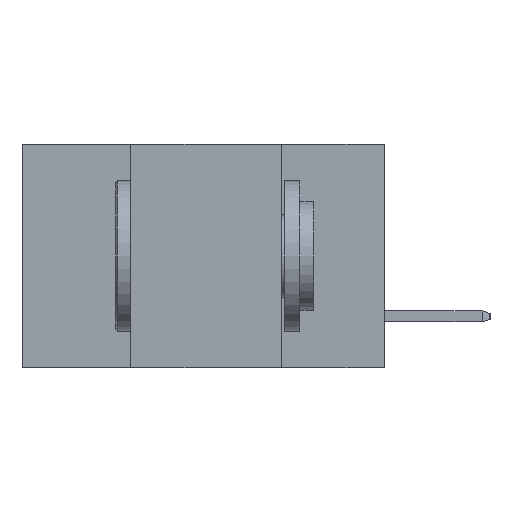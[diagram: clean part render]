
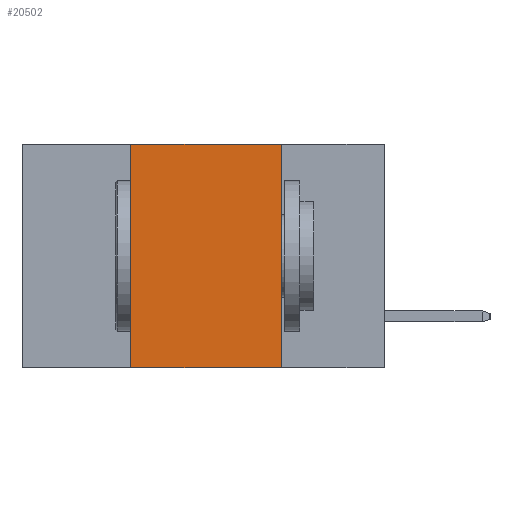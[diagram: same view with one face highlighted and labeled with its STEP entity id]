
A CAD part, left-side view. The second image highlights one B-rep face of the part: STEP entity #20502.
In plain terms, the highlighted planar face has unit normal (-1, 0, 0).
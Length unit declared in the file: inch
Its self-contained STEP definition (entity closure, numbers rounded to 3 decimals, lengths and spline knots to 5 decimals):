
#30 = DIRECTION ( 'NONE',  ( 0., 0., -1. ) ) ;
#224 = DIRECTION ( 'NONE',  ( 0., 0., 1. ) ) ;
#1218 = CARTESIAN_POINT ( 'NONE',  ( 0., 0.6, -0.37 ) ) ;
#2564 = LINE ( 'NONE', #15857, #6659 ) ;
#3887 = VERTEX_POINT ( 'NONE', #10185 ) ;
#6037 = EDGE_CURVE ( 'NONE', #11460, #7524, #2564, .T. ) ;
#6247 = CARTESIAN_POINT ( 'NONE',  ( 0., 0.17, -0.37 ) ) ;
#6659 = VECTOR ( 'NONE', #30, 39.37008 ) ;
#6867 = LINE ( 'NONE', #1218, #12126 ) ;
#7206 = ORIENTED_EDGE ( 'NONE', *, *, #8385, .F. ) ;
#7524 = VERTEX_POINT ( 'NONE', #6247 ) ;
#7824 = LINE ( 'NONE', #20864, #16975 ) ;
#8385 = EDGE_CURVE ( 'NONE', #17802, #11460, #7824, .T. ) ;
#9346 = DIRECTION ( 'NONE',  ( 0., -1., 0. ) ) ;
#10185 = CARTESIAN_POINT ( 'NONE',  ( 0., 0.42, -0.37 ) ) ;
#10246 = CARTESIAN_POINT ( 'NONE',  ( 0., 0.42, 0. ) ) ;
#11330 = FACE_OUTER_BOUND ( 'NONE', #12902, .T. ) ;
#11460 = VERTEX_POINT ( 'NONE', #13643 ) ;
#11835 = DIRECTION ( 'NONE',  ( 1., 0., 0. ) ) ;
#12126 = VECTOR ( 'NONE', #22686, 39.37008 ) ;
#12902 = EDGE_LOOP ( 'NONE', ( #16998, #7206, #14887, #19045 ) ) ;
#13643 = CARTESIAN_POINT ( 'NONE',  ( 0., 0.17, 0. ) ) ;
#14887 = ORIENTED_EDGE ( 'NONE', *, *, #24316, .F. ) ;
#15387 = VECTOR ( 'NONE', #224, 39.37008 ) ;
#15857 = CARTESIAN_POINT ( 'NONE',  ( 0., 0.17, 0. ) ) ;
#16975 = VECTOR ( 'NONE', #9346, 39.37008 ) ;
#16998 = ORIENTED_EDGE ( 'NONE', *, *, #6037, .F. ) ;
#17802 = VERTEX_POINT ( 'NONE', #18505 ) ;
#18505 = CARTESIAN_POINT ( 'NONE',  ( 0., 0.42, 0. ) ) ;
#18573 = AXIS2_PLACEMENT_3D ( 'NONE', #23291, #11835, #25206 ) ;
#19045 = ORIENTED_EDGE ( 'NONE', *, *, #23038, .T. ) ;
#19451 = PLANE ( 'NONE',  #18573 ) ;
#20502 = ADVANCED_FACE ( 'NONE', ( #11330 ), #19451, .F. ) ;
#20864 = CARTESIAN_POINT ( 'NONE',  ( 0., 0.6, 0. ) ) ;
#21031 = LINE ( 'NONE', #10246, #15387 ) ;
#22686 = DIRECTION ( 'NONE',  ( 0., -1., 0. ) ) ;
#23038 = EDGE_CURVE ( 'NONE', #3887, #7524, #6867, .T. ) ;
#23291 = CARTESIAN_POINT ( 'NONE',  ( 0., 0.6, 0. ) ) ;
#24316 = EDGE_CURVE ( 'NONE', #3887, #17802, #21031, .T. ) ;
#25206 = DIRECTION ( 'NONE',  ( 0., 0., -1. ) ) ;
